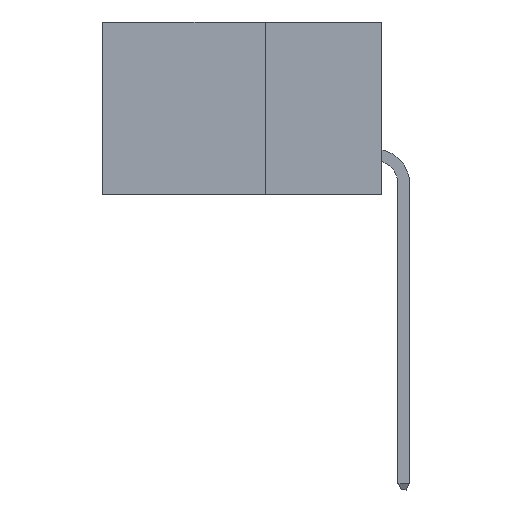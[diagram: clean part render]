
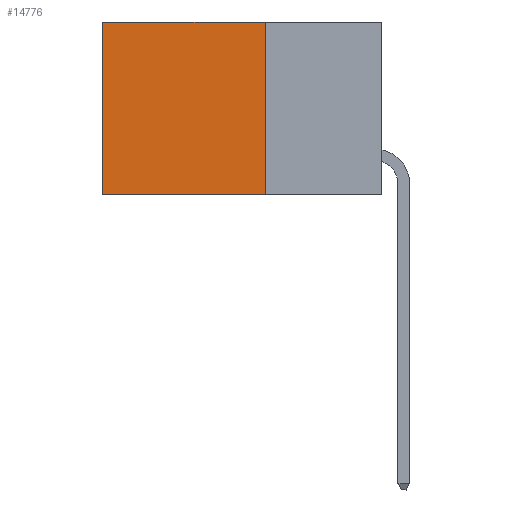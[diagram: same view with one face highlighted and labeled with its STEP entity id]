
A CAD part, left-side view. The second image highlights one B-rep face of the part: STEP entity #14776.
In plain terms, the highlighted planar face has unit normal (-1, 0, 0).
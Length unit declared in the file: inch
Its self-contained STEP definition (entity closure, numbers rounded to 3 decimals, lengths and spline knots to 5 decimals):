
#113 = CARTESIAN_POINT ( 'NONE',  ( 0.2875, 0.6, -0.37 ) ) ;
#650 = VECTOR ( 'NONE', #3825, 39.37008 ) ;
#1527 = EDGE_CURVE ( 'NONE', #7034, #7070, #3912, .T. ) ;
#1593 = ORIENTED_EDGE ( 'NONE', *, *, #12949, .F. ) ;
#1711 = DIRECTION ( 'NONE',  ( 1., 0., 0. ) ) ;
#3586 = CARTESIAN_POINT ( 'NONE',  ( 0.2875, 0.25, 0. ) ) ;
#3825 = DIRECTION ( 'NONE',  ( 0., 0., -1. ) ) ;
#3912 = LINE ( 'NONE', #8846, #650 ) ;
#4072 = VERTEX_POINT ( 'NONE', #13896 ) ;
#4096 = LINE ( 'NONE', #13915, #10328 ) ;
#4255 = DIRECTION ( 'NONE',  ( 0., 1., 0. ) ) ;
#5199 = EDGE_LOOP ( 'NONE', ( #14588, #1593, #10960, #6856 ) ) ;
#6701 = AXIS2_PLACEMENT_3D ( 'NONE', #10230, #1711, #8995 ) ;
#6856 = ORIENTED_EDGE ( 'NONE', *, *, #15712, .T. ) ;
#7034 = VERTEX_POINT ( 'NONE', #10648 ) ;
#7070 = VERTEX_POINT ( 'NONE', #11194 ) ;
#7161 = DIRECTION ( 'NONE',  ( 0., 1., 0. ) ) ;
#8514 = VECTOR ( 'NONE', #7161, 39.37008 ) ;
#8695 = CARTESIAN_POINT ( 'NONE',  ( 0.2875, 0.6, 0. ) ) ;
#8846 = CARTESIAN_POINT ( 'NONE',  ( 0.2875, 0.25, 0. ) ) ;
#8995 = DIRECTION ( 'NONE',  ( 0., 0., -1. ) ) ;
#10141 = FACE_OUTER_BOUND ( 'NONE', #5199, .T. ) ;
#10230 = CARTESIAN_POINT ( 'NONE',  ( 0.2875, 0.25, 0. ) ) ;
#10328 = VECTOR ( 'NONE', #4255, 39.37008 ) ;
#10648 = CARTESIAN_POINT ( 'NONE',  ( 0.2875, 0.25, 0. ) ) ;
#10826 = LINE ( 'NONE', #3586, #8514 ) ;
#10960 = ORIENTED_EDGE ( 'NONE', *, *, #1527, .F. ) ;
#11194 = CARTESIAN_POINT ( 'NONE',  ( 0.2875, 0.25, -0.37 ) ) ;
#11235 = DIRECTION ( 'NONE',  ( 0., 0., -1. ) ) ;
#12385 = VECTOR ( 'NONE', #11235, 39.37008 ) ;
#12949 = EDGE_CURVE ( 'NONE', #7070, #15003, #4096, .T. ) ;
#13896 = CARTESIAN_POINT ( 'NONE',  ( 0.2875, 0.6, 0. ) ) ;
#13915 = CARTESIAN_POINT ( 'NONE',  ( 0.2875, 0.25, -0.37 ) ) ;
#14185 = EDGE_CURVE ( 'NONE', #4072, #15003, #14805, .T. ) ;
#14588 = ORIENTED_EDGE ( 'NONE', *, *, #14185, .T. ) ;
#14776 = ADVANCED_FACE ( 'NONE', ( #10141 ), #15350, .F. ) ;
#14805 = LINE ( 'NONE', #8695, #12385 ) ;
#15003 = VERTEX_POINT ( 'NONE', #113 ) ;
#15350 = PLANE ( 'NONE',  #6701 ) ;
#15712 = EDGE_CURVE ( 'NONE', #7034, #4072, #10826, .T. ) ;
